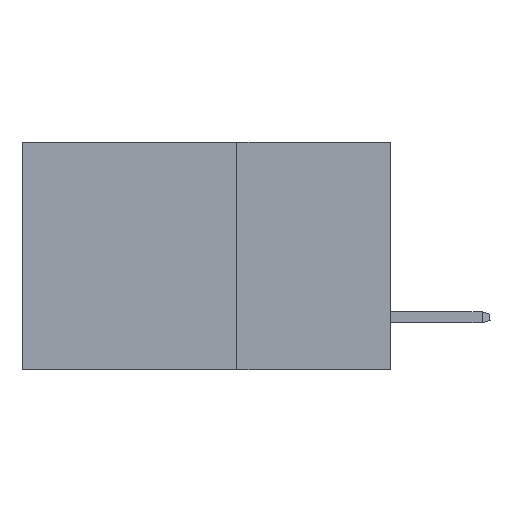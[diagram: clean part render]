
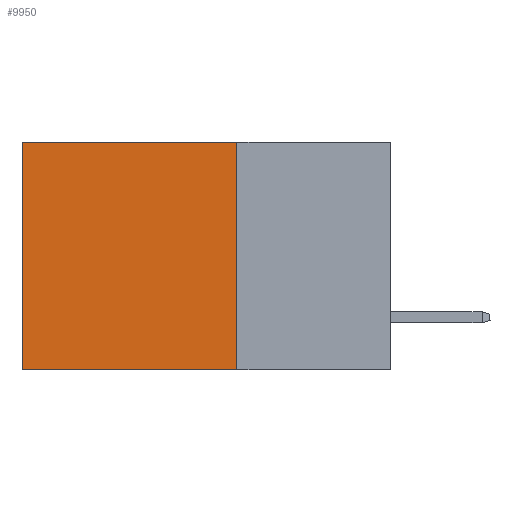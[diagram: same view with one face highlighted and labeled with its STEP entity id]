
A CAD part, left-side view. The second image highlights one B-rep face of the part: STEP entity #9950.
In plain terms, the highlighted planar face has unit normal (-1, 0, 0).
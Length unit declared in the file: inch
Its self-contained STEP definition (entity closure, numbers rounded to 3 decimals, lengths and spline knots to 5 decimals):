
#209 = FACE_OUTER_BOUND ( 'NONE', #2005, .T. ) ;
#2005 = EDGE_LOOP ( 'NONE', ( #34519, #10250, #21330, #19764 ) ) ;
#2538 = DIRECTION ( 'NONE',  ( 0., 0., -1. ) ) ;
#7305 = CARTESIAN_POINT ( 'NONE',  ( 0.2875, 0.25, 0. ) ) ;
#7799 = CARTESIAN_POINT ( 'NONE',  ( 0.2875, 0.25, -0.37 ) ) ;
#8982 = EDGE_CURVE ( 'NONE', #47553, #29163, #24241, .T. ) ;
#9950 = ADVANCED_FACE ( 'NONE', ( #209 ), #21288, .F. ) ;
#10250 = ORIENTED_EDGE ( 'NONE', *, *, #26937, .F. ) ;
#10340 = DIRECTION ( 'NONE',  ( 1., 0., 0. ) ) ;
#11584 = CARTESIAN_POINT ( 'NONE',  ( 0.2875, 0.6, 0. ) ) ;
#12346 = LINE ( 'NONE', #7799, #20534 ) ;
#15325 = DIRECTION ( 'NONE',  ( 0., 1., 0. ) ) ;
#19764 = ORIENTED_EDGE ( 'NONE', *, *, #42454, .T. ) ;
#20426 = VECTOR ( 'NONE', #25459, 39.37008 ) ;
#20534 = VECTOR ( 'NONE', #15325, 39.37008 ) ;
#21117 = CARTESIAN_POINT ( 'NONE',  ( 0.2875, 0.25, 0. ) ) ;
#21288 = PLANE ( 'NONE',  #41069 ) ;
#21330 = ORIENTED_EDGE ( 'NONE', *, *, #27746, .F. ) ;
#21457 = DIRECTION ( 'NONE',  ( 0., 0., -1. ) ) ;
#21912 = CARTESIAN_POINT ( 'NONE',  ( 0.2875, 0.6, -0.37 ) ) ;
#23096 = VECTOR ( 'NONE', #37717, 39.37008 ) ;
#24241 = LINE ( 'NONE', #11584, #23096 ) ;
#25459 = DIRECTION ( 'NONE',  ( 0., 1., 0. ) ) ;
#26937 = EDGE_CURVE ( 'NONE', #30397, #29163, #12346, .T. ) ;
#27746 = EDGE_CURVE ( 'NONE', #41504, #30397, #44447, .T. ) ;
#28028 = LINE ( 'NONE', #7305, #20426 ) ;
#28977 = CARTESIAN_POINT ( 'NONE',  ( 0.2875, 0.25, 0. ) ) ;
#29163 = VERTEX_POINT ( 'NONE', #21912 ) ;
#29308 = CARTESIAN_POINT ( 'NONE',  ( 0.2875, 0.25, -0.37 ) ) ;
#29791 = VECTOR ( 'NONE', #2538, 39.37008 ) ;
#30397 = VERTEX_POINT ( 'NONE', #29308 ) ;
#34519 = ORIENTED_EDGE ( 'NONE', *, *, #8982, .T. ) ;
#37717 = DIRECTION ( 'NONE',  ( 0., 0., -1. ) ) ;
#41069 = AXIS2_PLACEMENT_3D ( 'NONE', #28977, #10340, #21457 ) ;
#41504 = VERTEX_POINT ( 'NONE', #42881 ) ;
#42454 = EDGE_CURVE ( 'NONE', #41504, #47553, #28028, .T. ) ;
#42881 = CARTESIAN_POINT ( 'NONE',  ( 0.2875, 0.25, 0. ) ) ;
#44447 = LINE ( 'NONE', #21117, #29791 ) ;
#44821 = CARTESIAN_POINT ( 'NONE',  ( 0.2875, 0.6, 0. ) ) ;
#47553 = VERTEX_POINT ( 'NONE', #44821 ) ;
